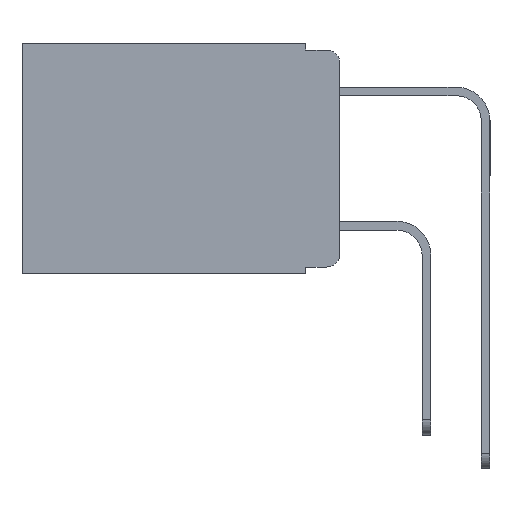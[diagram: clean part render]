
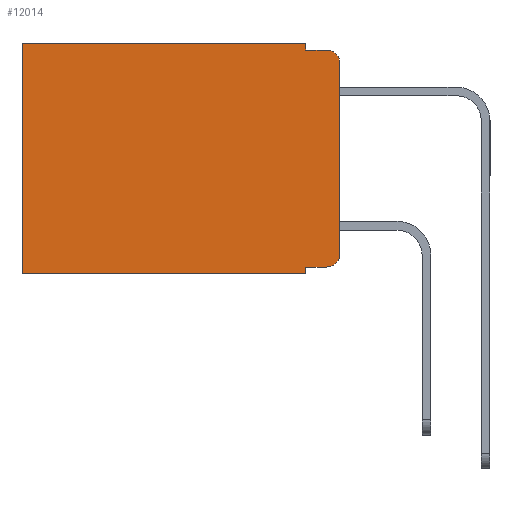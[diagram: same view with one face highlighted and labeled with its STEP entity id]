
A CAD part, left-side view. The second image highlights one B-rep face of the part: STEP entity #12014.
In plain terms, the highlighted planar face has unit normal (-1, 0, 0).
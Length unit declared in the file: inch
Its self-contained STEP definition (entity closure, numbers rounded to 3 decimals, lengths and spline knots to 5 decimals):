
#136 = ORIENTED_EDGE ( 'NONE', *, *, #14862, .F. ) ;
#199 = ORIENTED_EDGE ( 'NONE', *, *, #10151, .F. ) ;
#597 = DIRECTION ( 'NONE',  ( 0., 0., -1. ) ) ;
#695 = VERTEX_POINT ( 'NONE', #13695 ) ;
#945 = EDGE_CURVE ( 'NONE', #8285, #12900, #15683, .T. ) ;
#952 = DIRECTION ( 'NONE',  ( 0., 0., -1. ) ) ;
#1182 = CARTESIAN_POINT ( 'NONE',  ( 0.298, 0.02, -0.333 ) ) ;
#1376 = VECTOR ( 'NONE', #10888, 39.37008 ) ;
#1502 = ORIENTED_EDGE ( 'NONE', *, *, #12636, .T. ) ;
#1845 = ORIENTED_EDGE ( 'NONE', *, *, #7466, .T. ) ;
#2220 = LINE ( 'NONE', #4044, #12365 ) ;
#2268 = DIRECTION ( 'NONE',  ( -1., 0., 0. ) ) ;
#2379 = AXIS2_PLACEMENT_3D ( 'NONE', #15664, #15760, #15777 ) ;
#2541 = VECTOR ( 'NONE', #15344, 39.37008 ) ;
#2805 = DIRECTION ( 'NONE',  ( 0., 1., 0. ) ) ;
#3069 = ORIENTED_EDGE ( 'NONE', *, *, #15983, .F. ) ;
#3144 = VECTOR ( 'NONE', #3178, 39.37008 ) ;
#3178 = DIRECTION ( 'NONE',  ( 0., 0., -1. ) ) ;
#3635 = CARTESIAN_POINT ( 'NONE',  ( 0.298, 0.051, 0. ) ) ;
#3689 = CARTESIAN_POINT ( 'NONE',  ( 0.298, 0., -0.313 ) ) ;
#3778 = VERTEX_POINT ( 'NONE', #14367 ) ;
#3905 = VERTEX_POINT ( 'NONE', #12772 ) ;
#4044 = CARTESIAN_POINT ( 'NONE',  ( 0.298, 0.051, -0.01 ) ) ;
#4103 = AXIS2_PLACEMENT_3D ( 'NONE', #9812, #2268, #10978 ) ;
#4159 = VERTEX_POINT ( 'NONE', #10571 ) ;
#4989 = LINE ( 'NONE', #5989, #1376 ) ;
#5079 = VERTEX_POINT ( 'NONE', #1182 ) ;
#5141 = CARTESIAN_POINT ( 'NONE',  ( 0.298, 0.051, -0.333 ) ) ;
#5386 = DIRECTION ( 'NONE',  ( 0., 1., 0. ) ) ;
#5989 = CARTESIAN_POINT ( 'NONE',  ( 0.298, 0.473, 0. ) ) ;
#6398 = VERTEX_POINT ( 'NONE', #15869 ) ;
#6578 = VECTOR ( 'NONE', #5386, 39.37008 ) ;
#6750 = VECTOR ( 'NONE', #12073, 39.37008 ) ;
#6843 = LINE ( 'NONE', #12977, #2541 ) ;
#6950 = LINE ( 'NONE', #11326, #6578 ) ;
#7466 = EDGE_CURVE ( 'NONE', #5079, #12008, #14228, .T. ) ;
#7532 = PLANE ( 'NONE',  #10993 ) ;
#7757 = LINE ( 'NONE', #12792, #3144 ) ;
#8285 = VERTEX_POINT ( 'NONE', #9302 ) ;
#8349 = ORIENTED_EDGE ( 'NONE', *, *, #12367, .T. ) ;
#8580 = EDGE_CURVE ( 'NONE', #3778, #695, #4989, .T. ) ;
#8737 = DIRECTION ( 'NONE',  ( 1., 0., 0. ) ) ;
#9302 = CARTESIAN_POINT ( 'NONE',  ( 0.298, 0.051, 0. ) ) ;
#9812 = CARTESIAN_POINT ( 'NONE',  ( 0.298, 0.02, -0.03 ) ) ;
#10151 = EDGE_CURVE ( 'NONE', #15305, #3905, #12871, .T. ) ;
#10571 = CARTESIAN_POINT ( 'NONE',  ( 0.298, 0., -0.03 ) ) ;
#10598 = ORIENTED_EDGE ( 'NONE', *, *, #13636, .F. ) ;
#10888 = DIRECTION ( 'NONE',  ( 0., 0., -1. ) ) ;
#10978 = DIRECTION ( 'NONE',  ( 0., 0., -1. ) ) ;
#10993 = AXIS2_PLACEMENT_3D ( 'NONE', #15610, #8737, #952 ) ;
#11081 = EDGE_LOOP ( 'NONE', ( #10598, #15069, #3069, #15470, #8349, #11415, #136, #199, #1502, #1845 ) ) ;
#11326 = CARTESIAN_POINT ( 'NONE',  ( 0.298, 0., -0.343 ) ) ;
#11415 = ORIENTED_EDGE ( 'NONE', *, *, #8580, .T. ) ;
#11833 = CIRCLE ( 'NONE', #4103, 0.02 ) ;
#11933 = VECTOR ( 'NONE', #2805, 39.37008 ) ;
#12008 = VERTEX_POINT ( 'NONE', #3689 ) ;
#12014 = ADVANCED_FACE ( 'NONE', ( #15018 ), #7532, .F. ) ;
#12073 = DIRECTION ( 'NONE',  ( 0., 0., -1. ) ) ;
#12365 = VECTOR ( 'NONE', #12390, 39.37008 ) ;
#12367 = EDGE_CURVE ( 'NONE', #8285, #3778, #15002, .T. ) ;
#12390 = DIRECTION ( 'NONE',  ( 0., -1., 0. ) ) ;
#12555 = VECTOR ( 'NONE', #597, 39.37008 ) ;
#12636 = EDGE_CURVE ( 'NONE', #15305, #5079, #6843, .T. ) ;
#12772 = CARTESIAN_POINT ( 'NONE',  ( 0.298, 0.051, -0.343 ) ) ;
#12792 = CARTESIAN_POINT ( 'NONE',  ( 0.298, 0., 0. ) ) ;
#12871 = LINE ( 'NONE', #3635, #6750 ) ;
#12900 = VERTEX_POINT ( 'NONE', #15994 ) ;
#12977 = CARTESIAN_POINT ( 'NONE',  ( 0.298, 0.051, -0.333 ) ) ;
#13584 = CARTESIAN_POINT ( 'NONE',  ( 0.298, 0.051, 0. ) ) ;
#13636 = EDGE_CURVE ( 'NONE', #4159, #12008, #7757, .T. ) ;
#13695 = CARTESIAN_POINT ( 'NONE',  ( 0.298, 0.473, -0.343 ) ) ;
#14228 = CIRCLE ( 'NONE', #2379, 0.02 ) ;
#14367 = CARTESIAN_POINT ( 'NONE',  ( 0.298, 0.473, 0. ) ) ;
#14775 = CARTESIAN_POINT ( 'NONE',  ( 0.298, 0., 0. ) ) ;
#14862 = EDGE_CURVE ( 'NONE', #3905, #695, #6950, .T. ) ;
#15002 = LINE ( 'NONE', #14775, #11933 ) ;
#15018 = FACE_OUTER_BOUND ( 'NONE', #11081, .T. ) ;
#15069 = ORIENTED_EDGE ( 'NONE', *, *, #15201, .T. ) ;
#15201 = EDGE_CURVE ( 'NONE', #4159, #6398, #11833, .T. ) ;
#15305 = VERTEX_POINT ( 'NONE', #5141 ) ;
#15344 = DIRECTION ( 'NONE',  ( 0., -1., 0. ) ) ;
#15470 = ORIENTED_EDGE ( 'NONE', *, *, #945, .F. ) ;
#15610 = CARTESIAN_POINT ( 'NONE',  ( 0.298, 0., 0. ) ) ;
#15664 = CARTESIAN_POINT ( 'NONE',  ( 0.298, 0.02, -0.313 ) ) ;
#15683 = LINE ( 'NONE', #13584, #12555 ) ;
#15760 = DIRECTION ( 'NONE',  ( -1., 0., 0. ) ) ;
#15777 = DIRECTION ( 'NONE',  ( 0., 0., -1. ) ) ;
#15869 = CARTESIAN_POINT ( 'NONE',  ( 0.298, 0.02, -0.01 ) ) ;
#15983 = EDGE_CURVE ( 'NONE', #12900, #6398, #2220, .T. ) ;
#15994 = CARTESIAN_POINT ( 'NONE',  ( 0.298, 0.051, -0.01 ) ) ;
